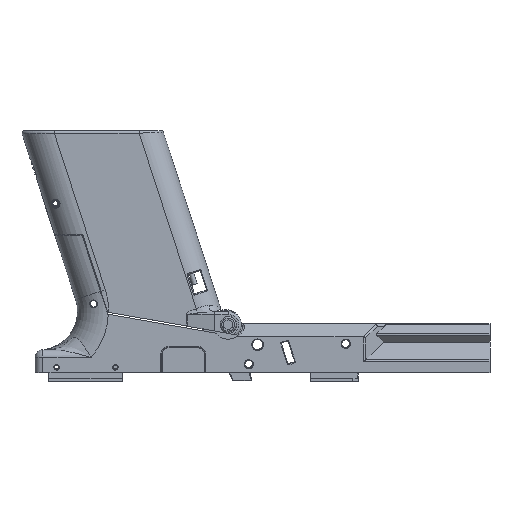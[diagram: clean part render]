
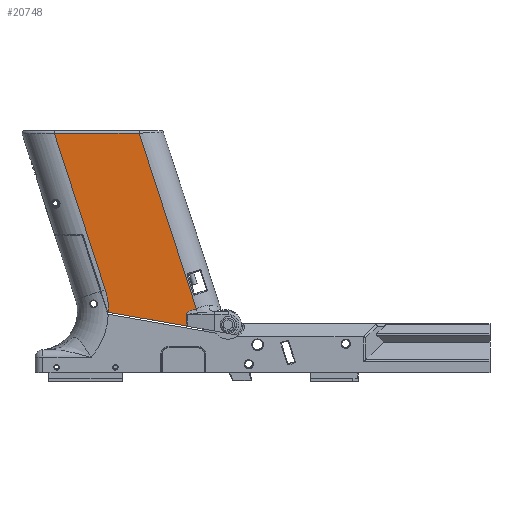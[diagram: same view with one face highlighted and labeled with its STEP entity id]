
A CAD part, front view. The second image highlights one B-rep face of the part: STEP entity #20748.
In plain terms, the highlighted planar face has unit normal (0, -1, 0).
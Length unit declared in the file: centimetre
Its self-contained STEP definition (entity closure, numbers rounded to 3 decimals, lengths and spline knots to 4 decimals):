
#328=ELLIPSE($,#22992,2.1378,0.4);
#674=PLANE($,#22991);
#2232=CIRCLE($,#22915,2.7);
#3588=FACE_OUTER_BOUND($,#4986,.T.);
#4986=EDGE_LOOP($,(#18483,#18484,#18485,#18486,#18487,#18488,#18489));
#6762=LINE($,#38949,#8164);
#6836=LINE($,#39795,#8238);
#6841=LINE($,#40137,#8243);
#6842=LINE($,#40147,#8244);
#6843=LINE($,#40149,#8245);
#8164=VECTOR($,#28323,3.0692);
#8238=VECTOR($,#28553,3.2918);
#8243=VECTOR($,#28590,7.1645);
#8244=VECTOR($,#28595,0.4466);
#8245=VECTOR($,#28598,6.3853);
#9896=VERTEX_POINT($,#38947);
#9897=VERTEX_POINT($,#38948);
#9932=VERTEX_POINT($,#39078);
#10009=VERTEX_POINT($,#39791);
#10010=VERTEX_POINT($,#39793);
#10046=VERTEX_POINT($,#40136);
#10048=VERTEX_POINT($,#40146);
#12700=EDGE_CURVE($,#9896,#9897,#6762,.T.);
#12744=EDGE_CURVE($,#9896,#9932,#2232,.T.);
#12865=EDGE_CURVE($,#10010,#10009,#6836,.T.);
#12910=EDGE_CURVE($,#10046,#10009,#6841,.T.);
#12913=EDGE_CURVE($,#10048,#9897,#6842,.T.);
#12914=EDGE_CURVE($,#10046,#10048,#328,.T.);
#12915=EDGE_CURVE($,#9932,#10010,#6843,.T.);
#18483=ORIENTED_EDGE($,*,*,#12700,.T.);
#18484=ORIENTED_EDGE($,*,*,#12913,.F.);
#18485=ORIENTED_EDGE($,*,*,#12914,.F.);
#18486=ORIENTED_EDGE($,*,*,#12910,.T.);
#18487=ORIENTED_EDGE($,*,*,#12865,.F.);
#18488=ORIENTED_EDGE($,*,*,#12915,.F.);
#18489=ORIENTED_EDGE($,*,*,#12744,.F.);
#20748=ADVANCED_FACE($,(#3588),#674,.F.);
#22915=AXIS2_PLACEMENT_3D($,#39079,#28383,#28384);
#22991=AXIS2_PLACEMENT_3D($,#40145,#28593,#28594);
#22992=AXIS2_PLACEMENT_3D($,#40148,#28596,#28597);
#28323=DIRECTION($,(0.985,0.,-0.174));
#28383=DIRECTION('center_axis',(0.,-1.,0.));
#28384=DIRECTION('ref_axis',(0.891,0.,-0.454));
#28553=DIRECTION($,(1.,0.,0.));
#28590=DIRECTION($,(-0.309,0.,0.951));
#28593=DIRECTION('center_axis',(0.,1.,0.));
#28594=DIRECTION('ref_axis',(0.,0.,1.));
#28595=DIRECTION($,(0.,0.,-1.));
#28596=DIRECTION('center_axis',(0.,-1.,0.));
#28597=DIRECTION('ref_axis',(-1.,0.,0.));
#28598=DIRECTION($,(-0.309,0.,0.951));
#38947=CARTESIAN_POINT('',(-5.2637,8.445,-1.6797));
#38948=CARTESIAN_POINT('',(-2.2411,8.445,-2.2127));
#38949=CARTESIAN_POINT($,(-3.8706,8.445,-1.9254));
#39078=CARTESIAN_POINT('',(-5.3954,8.445,-0.7979));
#39079=CARTESIAN_POINT('Origin',(-7.9632,8.445,-1.6323));
#39791=CARTESIAN_POINT('',(-4.0768,8.445,5.2749));
#39793=CARTESIAN_POINT('',(-7.3686,8.445,5.2749));
#39795=CARTESIAN_POINT($,(-1.8185,8.445,5.2749));
#40136=CARTESIAN_POINT('',(-1.8629,8.445,-1.5389));
#40137=CARTESIAN_POINT($,(-2.7394,8.445,1.1589));
#40145=CARTESIAN_POINT('Origin',(-4.5554,8.445,-3.0161));
#40146=CARTESIAN_POINT('',(-2.2411,8.445,-1.7661));
#40147=CARTESIAN_POINT($,(-2.2411,8.445,-2.5916));
#40148=CARTESIAN_POINT('Origin',(-0.1033,8.445,-1.7661));
#40149=CARTESIAN_POINT($,(-6.0027,8.445,1.0713));
